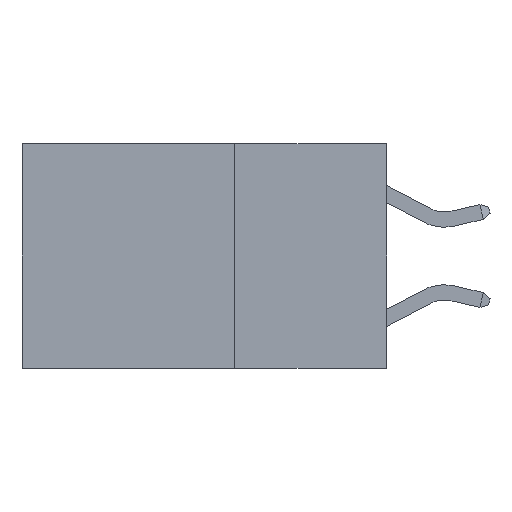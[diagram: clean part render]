
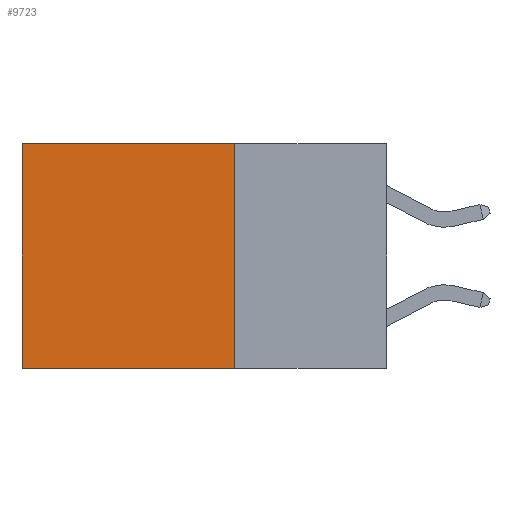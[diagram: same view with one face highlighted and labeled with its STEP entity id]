
A CAD part, left-side view. The second image highlights one B-rep face of the part: STEP entity #9723.
In plain terms, the highlighted planar face has unit normal (-1, 0, 0).
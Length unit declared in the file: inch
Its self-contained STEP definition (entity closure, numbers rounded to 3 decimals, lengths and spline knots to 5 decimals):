
#1114 = DIRECTION ( 'NONE',  ( 0., 1., 0. ) ) ;
#1858 = ORIENTED_EDGE ( 'NONE', *, *, #10359, .F. ) ;
#2697 = CARTESIAN_POINT ( 'NONE',  ( 0.2625, 0.6, 0. ) ) ;
#3827 = VECTOR ( 'NONE', #14305, 39.37008 ) ;
#4304 = LINE ( 'NONE', #22439, #8692 ) ;
#5752 = PLANE ( 'NONE',  #11092 ) ;
#6972 = CARTESIAN_POINT ( 'NONE',  ( 0.2625, 0.25, -0.37 ) ) ;
#7415 = DIRECTION ( 'NONE',  ( 1., 0., 0. ) ) ;
#8623 = ORIENTED_EDGE ( 'NONE', *, *, #11669, .F. ) ;
#8692 = VECTOR ( 'NONE', #11641, 39.37008 ) ;
#9723 = ADVANCED_FACE ( 'NONE', ( #21754 ), #5752, .F. ) ;
#9883 = DIRECTION ( 'NONE',  ( 0., 0., -1. ) ) ;
#10193 = CARTESIAN_POINT ( 'NONE',  ( 0.2625, 0.25, 0. ) ) ;
#10306 = CARTESIAN_POINT ( 'NONE',  ( 0.2625, 0.6, -0.37 ) ) ;
#10359 = EDGE_CURVE ( 'NONE', #21097, #13109, #15965, .T. ) ;
#11092 = AXIS2_PLACEMENT_3D ( 'NONE', #19968, #7415, #14624 ) ;
#11641 = DIRECTION ( 'NONE',  ( 0., 0., -1. ) ) ;
#11669 = EDGE_CURVE ( 'NONE', #12841, #21097, #4304, .T. ) ;
#11693 = EDGE_CURVE ( 'NONE', #12841, #12868, #23142, .T. ) ;
#12841 = VERTEX_POINT ( 'NONE', #21970 ) ;
#12868 = VERTEX_POINT ( 'NONE', #16524 ) ;
#13109 = VERTEX_POINT ( 'NONE', #10306 ) ;
#13240 = VECTOR ( 'NONE', #1114, 39.37008 ) ;
#14305 = DIRECTION ( 'NONE',  ( 0., 1., 0. ) ) ;
#14624 = DIRECTION ( 'NONE',  ( 0., 0., -1. ) ) ;
#15965 = LINE ( 'NONE', #6972, #3827 ) ;
#16524 = CARTESIAN_POINT ( 'NONE',  ( 0.2625, 0.6, 0. ) ) ;
#16985 = EDGE_CURVE ( 'NONE', #12868, #13109, #22606, .T. ) ;
#19114 = VECTOR ( 'NONE', #9883, 39.37008 ) ;
#19968 = CARTESIAN_POINT ( 'NONE',  ( 0.2625, 0.25, 0. ) ) ;
#21097 = VERTEX_POINT ( 'NONE', #22395 ) ;
#21754 = FACE_OUTER_BOUND ( 'NONE', #23243, .T. ) ;
#21914 = ORIENTED_EDGE ( 'NONE', *, *, #16985, .T. ) ;
#21970 = CARTESIAN_POINT ( 'NONE',  ( 0.2625, 0.25, 0. ) ) ;
#22395 = CARTESIAN_POINT ( 'NONE',  ( 0.2625, 0.25, -0.37 ) ) ;
#22439 = CARTESIAN_POINT ( 'NONE',  ( 0.2625, 0.25, 0. ) ) ;
#22606 = LINE ( 'NONE', #2697, #19114 ) ;
#23053 = ORIENTED_EDGE ( 'NONE', *, *, #11693, .T. ) ;
#23142 = LINE ( 'NONE', #10193, #13240 ) ;
#23243 = EDGE_LOOP ( 'NONE', ( #21914, #1858, #8623, #23053 ) ) ;
